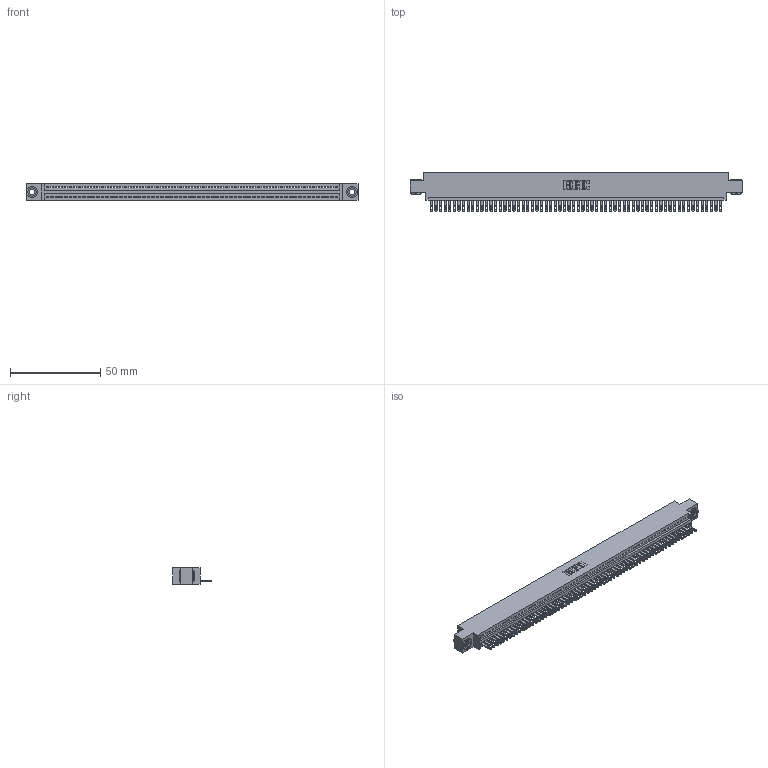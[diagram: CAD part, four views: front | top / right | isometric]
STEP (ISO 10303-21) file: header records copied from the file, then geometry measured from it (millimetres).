
FILE_DESCRIPTION (( 'STEP AP203' ), '1' );
FILE_NAME ('895-064-500-603.STEP', '2020-09-28T09:57:06', ( '' ), ( '' ), 'SwSTEP 2.0', 'SolidWorks 2020', '' );
FILE_SCHEMA (( 'CONFIG_CONTROL_DESIGN' ));
Length unit declared in the file: inch
Products named in the file (4): 345-250-002_345-250-002-102; 845 Part_0.170 Offset - 0.156 Dia-TH; 895-064-500-603; 345-292-001_345-293-100
Assembly tree (67 placements, depth 2):
  895-064-500-603
    845 Part_0.170 Offset - 0.156 Dia-TH
    345-292-001_345-293-100  x64
    345-250-002_345-250-002-102  x2
Bounding box: 183.77 x 21.51 x 9.4 mm (x, y, z)
Volume: 17580.4 mm3; surface area: 24146.5 mm2
Topology: 67 solids, 67 shells, 3624 faces, 11181 edges, 7450 vertices
Faces by surface type: plane 2270, cylinder 1346, cone 8
Entity records: 45918 total; most frequent: CARTESIAN_POINT 7931, ORIENTED_EDGE 7922, DIRECTION 6927, EDGE_CURVE 3961, LINE 3545, VECTOR 3545, VERTEX_POINT 2638, AXIS2_PLACEMENT_3D 1691
